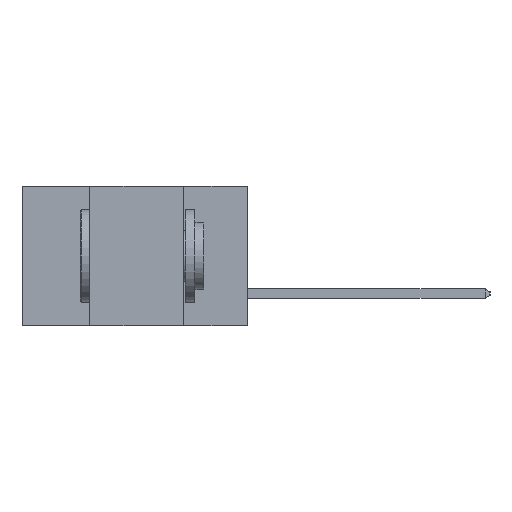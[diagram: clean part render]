
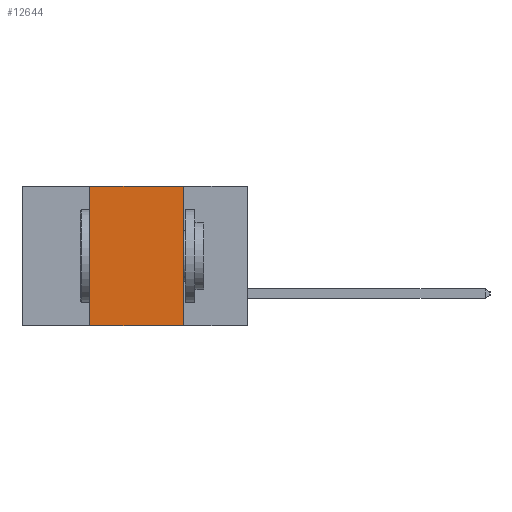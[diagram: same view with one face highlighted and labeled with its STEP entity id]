
A CAD part, left-side view. The second image highlights one B-rep face of the part: STEP entity #12644.
In plain terms, the highlighted planar face has unit normal (-1, 0, 0).
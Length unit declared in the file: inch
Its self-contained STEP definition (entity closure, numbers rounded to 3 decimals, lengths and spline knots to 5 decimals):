
#46 = CARTESIAN_POINT ( 'NONE',  ( 0., 0.42, -0.37 ) ) ;
#451 = DIRECTION ( 'NONE',  ( 0., 0., -1. ) ) ;
#920 = CARTESIAN_POINT ( 'NONE',  ( 0., 0.17, 0. ) ) ;
#1444 = VERTEX_POINT ( 'NONE', #46 ) ;
#2664 = EDGE_CURVE ( 'NONE', #6654, #8768, #20596, .T. ) ;
#3671 = CARTESIAN_POINT ( 'NONE',  ( 0., 0.6, 0. ) ) ;
#5228 = VECTOR ( 'NONE', #14611, 39.37008 ) ;
#6149 = DIRECTION ( 'NONE',  ( 0., -1., 0. ) ) ;
#6636 = VECTOR ( 'NONE', #6149, 39.37008 ) ;
#6654 = VERTEX_POINT ( 'NONE', #32543 ) ;
#7760 = FACE_OUTER_BOUND ( 'NONE', #16948, .T. ) ;
#7852 = VECTOR ( 'NONE', #25832, 39.37008 ) ;
#8768 = VERTEX_POINT ( 'NONE', #19659 ) ;
#10399 = ORIENTED_EDGE ( 'NONE', *, *, #15374, .F. ) ;
#11650 = EDGE_CURVE ( 'NONE', #25999, #6654, #14307, .T. ) ;
#12644 = ADVANCED_FACE ( 'NONE', ( #7760 ), #18244, .F. ) ;
#13228 = LINE ( 'NONE', #18508, #30768 ) ;
#14307 = LINE ( 'NONE', #3671, #6636 ) ;
#14611 = DIRECTION ( 'NONE',  ( 0., 0., 1. ) ) ;
#15374 = EDGE_CURVE ( 'NONE', #1444, #25999, #17994, .T. ) ;
#15850 = DIRECTION ( 'NONE',  ( 1., 0., 0. ) ) ;
#16878 = AXIS2_PLACEMENT_3D ( 'NONE', #30705, #15850, #451 ) ;
#16948 = EDGE_LOOP ( 'NONE', ( #22880, #23309, #10399, #28889 ) ) ;
#17994 = LINE ( 'NONE', #27031, #5228 ) ;
#18244 = PLANE ( 'NONE',  #16878 ) ;
#18508 = CARTESIAN_POINT ( 'NONE',  ( 0., 0.6, -0.37 ) ) ;
#19659 = CARTESIAN_POINT ( 'NONE',  ( 0., 0.17, -0.37 ) ) ;
#20596 = LINE ( 'NONE', #920, #7852 ) ;
#21027 = DIRECTION ( 'NONE',  ( 0., -1., 0. ) ) ;
#22880 = ORIENTED_EDGE ( 'NONE', *, *, #2664, .F. ) ;
#23309 = ORIENTED_EDGE ( 'NONE', *, *, #11650, .F. ) ;
#23770 = CARTESIAN_POINT ( 'NONE',  ( 0., 0.42, 0. ) ) ;
#25832 = DIRECTION ( 'NONE',  ( 0., 0., -1. ) ) ;
#25999 = VERTEX_POINT ( 'NONE', #23770 ) ;
#27031 = CARTESIAN_POINT ( 'NONE',  ( 0., 0.42, 0. ) ) ;
#28889 = ORIENTED_EDGE ( 'NONE', *, *, #30957, .T. ) ;
#30705 = CARTESIAN_POINT ( 'NONE',  ( 0., 0.6, 0. ) ) ;
#30768 = VECTOR ( 'NONE', #21027, 39.37008 ) ;
#30957 = EDGE_CURVE ( 'NONE', #1444, #8768, #13228, .T. ) ;
#32543 = CARTESIAN_POINT ( 'NONE',  ( 0., 0.17, 0. ) ) ;
